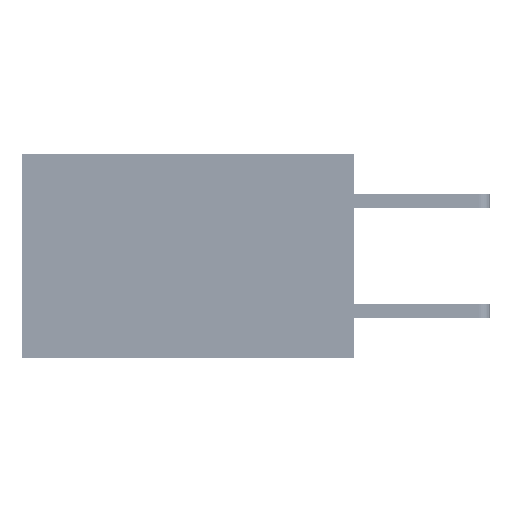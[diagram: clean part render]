
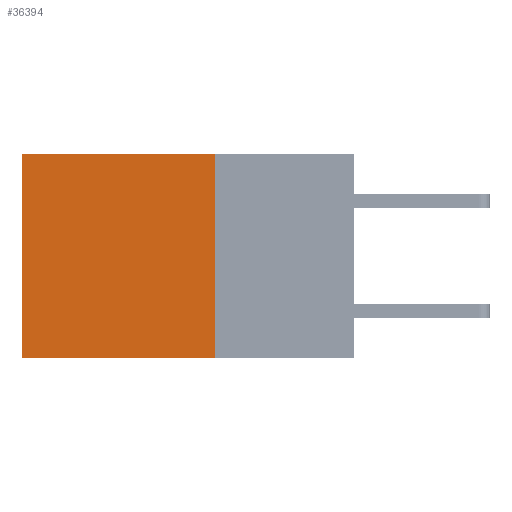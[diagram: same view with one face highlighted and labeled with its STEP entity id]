
A CAD part, left-side view. The second image highlights one B-rep face of the part: STEP entity #36394.
In plain terms, the highlighted planar face has unit normal (-1, 0, 0).
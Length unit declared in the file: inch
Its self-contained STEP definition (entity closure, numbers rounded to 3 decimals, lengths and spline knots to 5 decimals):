
#467 = ORIENTED_EDGE ( 'NONE', *, *, #21894, .T. ) ;
#2399 = AXIS2_PLACEMENT_3D ( 'NONE', #27504, #16170, #31458 ) ;
#3264 = CARTESIAN_POINT ( 'NONE',  ( 0.2875, 0.25, 0. ) ) ;
#3703 = PLANE ( 'NONE',  #2399 ) ;
#6305 = DIRECTION ( 'NONE',  ( 0., 1., 0. ) ) ;
#6678 = CARTESIAN_POINT ( 'NONE',  ( 0.2875, 0.25, 0. ) ) ;
#8595 = LINE ( 'NONE', #3264, #12896 ) ;
#9787 = CARTESIAN_POINT ( 'NONE',  ( 0.2875, 0.6, 0. ) ) ;
#11895 = LINE ( 'NONE', #32570, #34229 ) ;
#12896 = VECTOR ( 'NONE', #6305, 39.37008 ) ;
#13414 = ORIENTED_EDGE ( 'NONE', *, *, #24642, .F. ) ;
#13887 = LINE ( 'NONE', #26793, #36190 ) ;
#16170 = DIRECTION ( 'NONE',  ( 1., 0., 0. ) ) ;
#19424 = VERTEX_POINT ( 'NONE', #33517 ) ;
#19705 = FACE_OUTER_BOUND ( 'NONE', #26457, .T. ) ;
#21894 = EDGE_CURVE ( 'NONE', #19424, #23903, #8595, .T. ) ;
#23903 = VERTEX_POINT ( 'NONE', #9787 ) ;
#24642 = EDGE_CURVE ( 'NONE', #19424, #33447, #39397, .T. ) ;
#26457 = EDGE_LOOP ( 'NONE', ( #29550, #30763, #13414, #467 ) ) ;
#26793 = CARTESIAN_POINT ( 'NONE',  ( 0.2875, 0.6, 0. ) ) ;
#27504 = CARTESIAN_POINT ( 'NONE',  ( 0.2875, 0.25, 0. ) ) ;
#29212 = CARTESIAN_POINT ( 'NONE',  ( 0.2875, 0.6, -0.37 ) ) ;
#29265 = DIRECTION ( 'NONE',  ( 0., 1., 0. ) ) ;
#29550 = ORIENTED_EDGE ( 'NONE', *, *, #31035, .T. ) ;
#30763 = ORIENTED_EDGE ( 'NONE', *, *, #38747, .F. ) ;
#31035 = EDGE_CURVE ( 'NONE', #23903, #37939, #13887, .T. ) ;
#31128 = DIRECTION ( 'NONE',  ( 0., 0., -1. ) ) ;
#31458 = DIRECTION ( 'NONE',  ( 0., 0., -1. ) ) ;
#31805 = VECTOR ( 'NONE', #31128, 39.37008 ) ;
#32570 = CARTESIAN_POINT ( 'NONE',  ( 0.2875, 0.25, -0.37 ) ) ;
#33447 = VERTEX_POINT ( 'NONE', #36479 ) ;
#33517 = CARTESIAN_POINT ( 'NONE',  ( 0.2875, 0.25, 0. ) ) ;
#33544 = DIRECTION ( 'NONE',  ( 0., 0., -1. ) ) ;
#34229 = VECTOR ( 'NONE', #29265, 39.37008 ) ;
#36190 = VECTOR ( 'NONE', #33544, 39.37008 ) ;
#36394 = ADVANCED_FACE ( 'NONE', ( #19705 ), #3703, .F. ) ;
#36479 = CARTESIAN_POINT ( 'NONE',  ( 0.2875, 0.25, -0.37 ) ) ;
#37939 = VERTEX_POINT ( 'NONE', #29212 ) ;
#38747 = EDGE_CURVE ( 'NONE', #33447, #37939, #11895, .T. ) ;
#39397 = LINE ( 'NONE', #6678, #31805 ) ;
